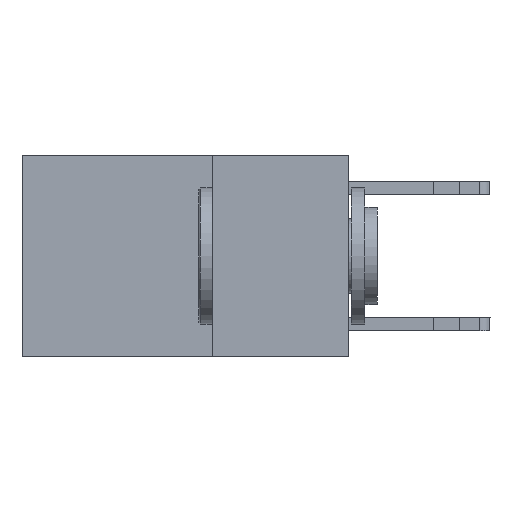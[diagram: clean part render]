
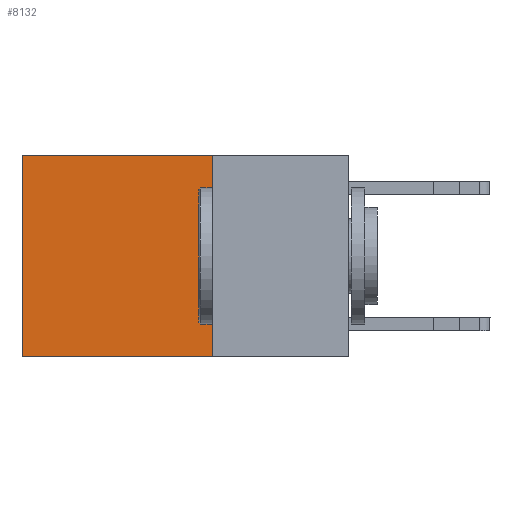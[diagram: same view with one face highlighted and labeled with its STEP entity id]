
A CAD part, left-side view. The second image highlights one B-rep face of the part: STEP entity #8132.
In plain terms, the highlighted planar face has unit normal (-1, 0, 0).
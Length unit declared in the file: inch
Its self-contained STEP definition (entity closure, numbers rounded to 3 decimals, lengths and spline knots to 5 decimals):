
#240 = VECTOR ( 'NONE', #5434, 39.37008 ) ;
#615 = ORIENTED_EDGE ( 'NONE', *, *, #11858, .T. ) ;
#617 = VERTEX_POINT ( 'NONE', #11859 ) ;
#679 = DIRECTION ( 'NONE',  ( 0., 1., 0. ) ) ;
#873 = CARTESIAN_POINT ( 'NONE',  ( 0.2625, 0.25, -0.37 ) ) ;
#1874 = LINE ( 'NONE', #6763, #11173 ) ;
#1914 = VECTOR ( 'NONE', #12980, 39.37008 ) ;
#2478 = FACE_OUTER_BOUND ( 'NONE', #4953, .T. ) ;
#3333 = CARTESIAN_POINT ( 'NONE',  ( 0.2625, 0.6, 0. ) ) ;
#4686 = PLANE ( 'NONE',  #11970 ) ;
#4953 = EDGE_LOOP ( 'NONE', ( #615, #15073, #7817, #14659 ) ) ;
#5156 = LINE ( 'NONE', #873, #1914 ) ;
#5285 = EDGE_CURVE ( 'NONE', #13299, #5388, #1874, .T. ) ;
#5388 = VERTEX_POINT ( 'NONE', #3333 ) ;
#5434 = DIRECTION ( 'NONE',  ( 0., 0., -1. ) ) ;
#5884 = CARTESIAN_POINT ( 'NONE',  ( 0.2625, 0.25, 0. ) ) ;
#6763 = CARTESIAN_POINT ( 'NONE',  ( 0.2625, 0.25, 0. ) ) ;
#7127 = DIRECTION ( 'NONE',  ( 0., 0., -1. ) ) ;
#7504 = DIRECTION ( 'NONE',  ( 0., 0., -1. ) ) ;
#7817 = ORIENTED_EDGE ( 'NONE', *, *, #12315, .F. ) ;
#8132 = ADVANCED_FACE ( 'NONE', ( #2478 ), #4686, .F. ) ;
#9042 = VERTEX_POINT ( 'NONE', #12282 ) ;
#9955 = LINE ( 'NONE', #10232, #240 ) ;
#10232 = CARTESIAN_POINT ( 'NONE',  ( 0.2625, 0.6, 0. ) ) ;
#11173 = VECTOR ( 'NONE', #679, 39.37008 ) ;
#11858 = EDGE_CURVE ( 'NONE', #5388, #9042, #9955, .T. ) ;
#11859 = CARTESIAN_POINT ( 'NONE',  ( 0.2625, 0.25, -0.37 ) ) ;
#11970 = AXIS2_PLACEMENT_3D ( 'NONE', #5884, #14245, #7127 ) ;
#12017 = VECTOR ( 'NONE', #7504, 39.37008 ) ;
#12282 = CARTESIAN_POINT ( 'NONE',  ( 0.2625, 0.6, -0.37 ) ) ;
#12315 = EDGE_CURVE ( 'NONE', #13299, #617, #14757, .T. ) ;
#12980 = DIRECTION ( 'NONE',  ( 0., 1., 0. ) ) ;
#13299 = VERTEX_POINT ( 'NONE', #13985 ) ;
#13439 = CARTESIAN_POINT ( 'NONE',  ( 0.2625, 0.25, 0. ) ) ;
#13985 = CARTESIAN_POINT ( 'NONE',  ( 0.2625, 0.25, 0. ) ) ;
#14102 = EDGE_CURVE ( 'NONE', #617, #9042, #5156, .T. ) ;
#14245 = DIRECTION ( 'NONE',  ( 1., 0., 0. ) ) ;
#14659 = ORIENTED_EDGE ( 'NONE', *, *, #5285, .T. ) ;
#14757 = LINE ( 'NONE', #13439, #12017 ) ;
#15073 = ORIENTED_EDGE ( 'NONE', *, *, #14102, .F. ) ;
